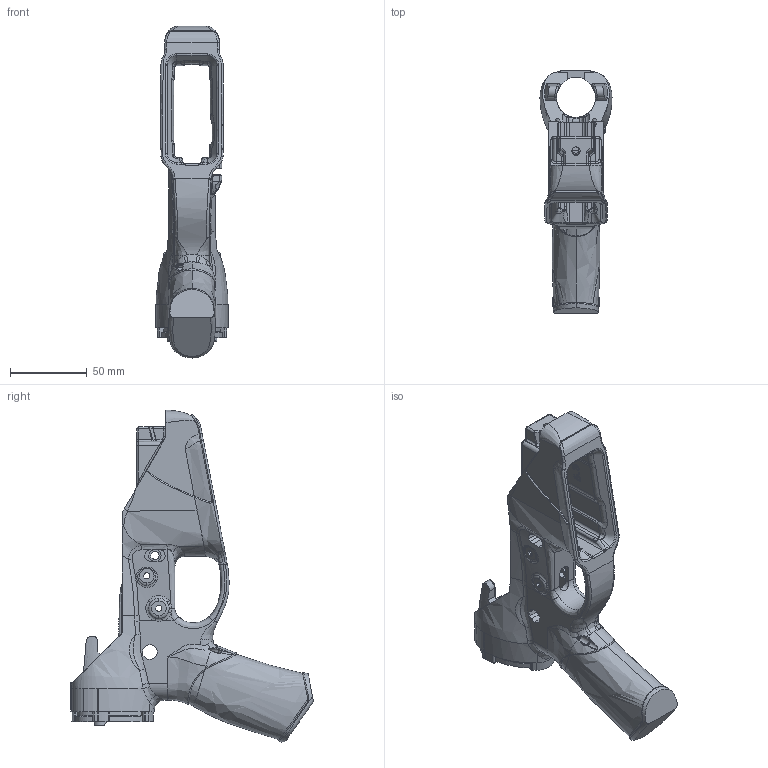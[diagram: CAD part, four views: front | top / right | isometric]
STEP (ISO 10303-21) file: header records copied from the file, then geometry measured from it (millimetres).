
FILE_DESCRIPTION (( 'STEP AP203' ), '1' );
FILE_NAME ('Orca Lower V5.3.STEP', '2023-01-20T23:40:35', ( '' ), ( '' ), 'SwSTEP 2.0', 'SolidWorks 2021', '' );
FILE_SCHEMA (( 'CONFIG_CONTROL_DESIGN' ));
Products named in the file (1): Orca Lower V5.3
Bounding box: 46.99 x 158.47 x 216.64 mm (x, y, z)
Volume: 264432 mm3; surface area: 68504.4 mm2
Topology: 1 solids, 1 shells, 905 faces, 2404 edges, 1486 vertices
Faces by surface type: bspline 424, cylinder 229, plane 186, torus 47, sphere 14, cone 5
Entity records: 82689 total; most frequent: CARTESIAN_POINT 63711, ORIENTED_EDGE 4762, DIRECTION 2845, EDGE_CURVE 2381, VERTEX_POINT 1486, AXIS2_PLACEMENT_3D 1077, B_SPLINE_CURVE_WITH_KNOTS 958, EDGE_LOOP 945
